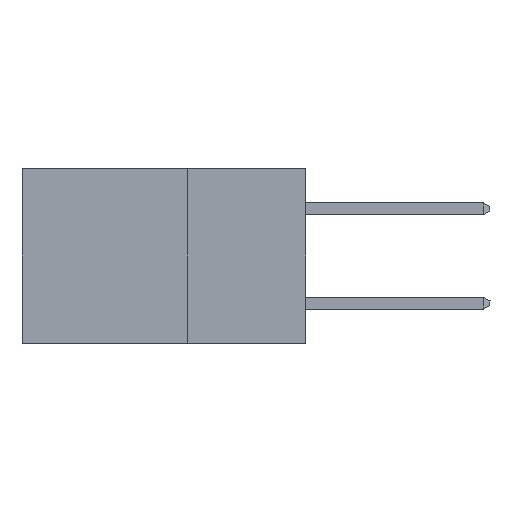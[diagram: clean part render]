
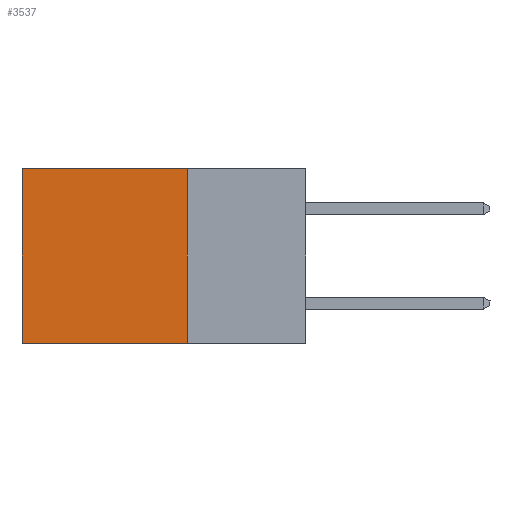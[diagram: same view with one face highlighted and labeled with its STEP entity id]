
A CAD part, left-side view. The second image highlights one B-rep face of the part: STEP entity #3537.
In plain terms, the highlighted planar face has unit normal (-1, 0, 0).
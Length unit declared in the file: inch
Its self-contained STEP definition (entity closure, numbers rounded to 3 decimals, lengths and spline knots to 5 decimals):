
#652 = DIRECTION ( 'NONE',  ( 0., 0., -1. ) ) ;
#930 = VECTOR ( 'NONE', #652, 39.37008 ) ;
#1391 = EDGE_LOOP ( 'NONE', ( #4575, #11426, #10755, #6842 ) ) ;
#1509 = CARTESIAN_POINT ( 'NONE',  ( 0.298, 0.25, -0.37 ) ) ;
#1864 = AXIS2_PLACEMENT_3D ( 'NONE', #2198, #2151, #13288 ) ;
#2151 = DIRECTION ( 'NONE',  ( 1., 0., 0. ) ) ;
#2198 = CARTESIAN_POINT ( 'NONE',  ( 0.298, 0.25, 0. ) ) ;
#3537 = ADVANCED_FACE ( 'NONE', ( #9341 ), #13185, .F. ) ;
#4575 = ORIENTED_EDGE ( 'NONE', *, *, #9661, .T. ) ;
#4668 = CARTESIAN_POINT ( 'NONE',  ( 0.298, 0.6, 0. ) ) ;
#4992 = VERTEX_POINT ( 'NONE', #4668 ) ;
#6102 = VECTOR ( 'NONE', #8743, 39.37008 ) ;
#6107 = CARTESIAN_POINT ( 'NONE',  ( 0.298, 0.25, -0.37 ) ) ;
#6119 = VERTEX_POINT ( 'NONE', #6107 ) ;
#6337 = CARTESIAN_POINT ( 'NONE',  ( 0.298, 0.25, 0. ) ) ;
#6842 = ORIENTED_EDGE ( 'NONE', *, *, #9201, .T. ) ;
#7007 = LINE ( 'NONE', #1509, #7954 ) ;
#7360 = VERTEX_POINT ( 'NONE', #6337 ) ;
#7908 = CARTESIAN_POINT ( 'NONE',  ( 0.298, 0.25, 0. ) ) ;
#7954 = VECTOR ( 'NONE', #11463, 39.37008 ) ;
#8272 = CARTESIAN_POINT ( 'NONE',  ( 0.298, 0.6, -0.37 ) ) ;
#8353 = LINE ( 'NONE', #15006, #10642 ) ;
#8596 = VERTEX_POINT ( 'NONE', #8272 ) ;
#8743 = DIRECTION ( 'NONE',  ( 0., 0., -1. ) ) ;
#9201 = EDGE_CURVE ( 'NONE', #7360, #4992, #8353, .T. ) ;
#9341 = FACE_OUTER_BOUND ( 'NONE', #1391, .T. ) ;
#9508 = LINE ( 'NONE', #11128, #6102 ) ;
#9661 = EDGE_CURVE ( 'NONE', #4992, #8596, #9508, .T. ) ;
#10642 = VECTOR ( 'NONE', #15525, 39.37008 ) ;
#10755 = ORIENTED_EDGE ( 'NONE', *, *, #10948, .F. ) ;
#10774 = EDGE_CURVE ( 'NONE', #6119, #8596, #7007, .T. ) ;
#10948 = EDGE_CURVE ( 'NONE', #7360, #6119, #13927, .T. ) ;
#11128 = CARTESIAN_POINT ( 'NONE',  ( 0.298, 0.6, 0. ) ) ;
#11426 = ORIENTED_EDGE ( 'NONE', *, *, #10774, .F. ) ;
#11463 = DIRECTION ( 'NONE',  ( 0., 1., 0. ) ) ;
#13185 = PLANE ( 'NONE',  #1864 ) ;
#13288 = DIRECTION ( 'NONE',  ( 0., 0., -1. ) ) ;
#13927 = LINE ( 'NONE', #7908, #930 ) ;
#15006 = CARTESIAN_POINT ( 'NONE',  ( 0.298, 0.25, 0. ) ) ;
#15525 = DIRECTION ( 'NONE',  ( 0., 1., 0. ) ) ;
